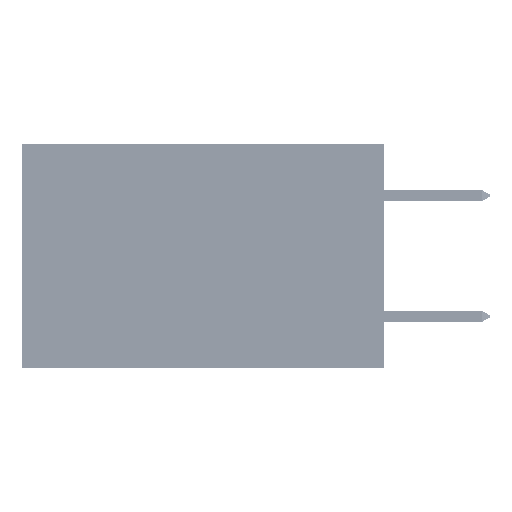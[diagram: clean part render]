
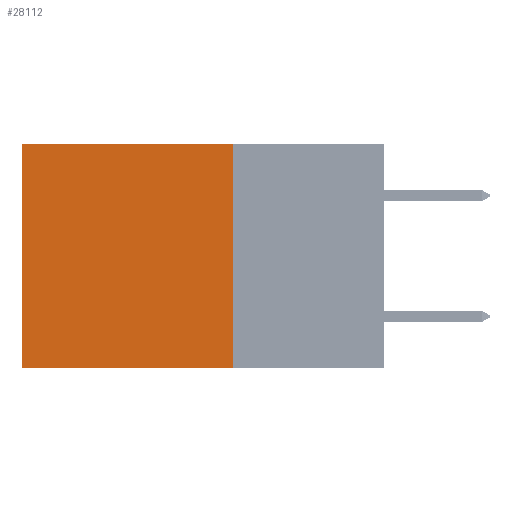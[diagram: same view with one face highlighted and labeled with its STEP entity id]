
A CAD part, left-side view. The second image highlights one B-rep face of the part: STEP entity #28112.
In plain terms, the highlighted planar face has unit normal (-1, 0, 0).
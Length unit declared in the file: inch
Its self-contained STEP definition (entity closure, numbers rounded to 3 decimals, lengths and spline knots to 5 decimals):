
#1281 = CARTESIAN_POINT ( 'NONE',  ( 0.2875, 0.25, 0. ) ) ;
#1449 = VECTOR ( 'NONE', #10237, 39.37008 ) ;
#1700 = FACE_OUTER_BOUND ( 'NONE', #33100, .T. ) ;
#1906 = CARTESIAN_POINT ( 'NONE',  ( 0.2875, 0.25, 0. ) ) ;
#2276 = DIRECTION ( 'NONE',  ( 0., 1., 0. ) ) ;
#2353 = EDGE_CURVE ( 'NONE', #35352, #40141, #32204, .T. ) ;
#5336 = ORIENTED_EDGE ( 'NONE', *, *, #24309, .F. ) ;
#5429 = DIRECTION ( 'NONE',  ( 0., 0., -1. ) ) ;
#9925 = VECTOR ( 'NONE', #2276, 39.37008 ) ;
#10237 = DIRECTION ( 'NONE',  ( 0., 0., -1. ) ) ;
#12402 = ORIENTED_EDGE ( 'NONE', *, *, #31972, .T. ) ;
#12416 = CARTESIAN_POINT ( 'NONE',  ( 0.2875, 0.6, 0. ) ) ;
#12793 = VERTEX_POINT ( 'NONE', #1906 ) ;
#14667 = CARTESIAN_POINT ( 'NONE',  ( 0.2875, 0.6, -0.37 ) ) ;
#14896 = CARTESIAN_POINT ( 'NONE',  ( 0.2875, 0.25, 0. ) ) ;
#17200 = PLANE ( 'NONE',  #48892 ) ;
#18864 = DIRECTION ( 'NONE',  ( 0., 1., 0. ) ) ;
#20450 = LINE ( 'NONE', #37939, #40270 ) ;
#23690 = LINE ( 'NONE', #29951, #1449 ) ;
#24309 = EDGE_CURVE ( 'NONE', #12793, #35352, #23690, .T. ) ;
#25764 = LINE ( 'NONE', #14896, #45591 ) ;
#28112 = ADVANCED_FACE ( 'NONE', ( #1700 ), #17200, .F. ) ;
#28723 = EDGE_CURVE ( 'NONE', #12793, #43951, #25764, .T. ) ;
#29095 = DIRECTION ( 'NONE',  ( 1., 0., 0. ) ) ;
#29689 = ORIENTED_EDGE ( 'NONE', *, *, #2353, .F. ) ;
#29951 = CARTESIAN_POINT ( 'NONE',  ( 0.2875, 0.25, 0. ) ) ;
#31972 = EDGE_CURVE ( 'NONE', #43951, #40141, #20450, .T. ) ;
#32204 = LINE ( 'NONE', #45708, #9925 ) ;
#33100 = EDGE_LOOP ( 'NONE', ( #12402, #29689, #5336, #33393 ) ) ;
#33393 = ORIENTED_EDGE ( 'NONE', *, *, #28723, .T. ) ;
#35352 = VERTEX_POINT ( 'NONE', #46713 ) ;
#37939 = CARTESIAN_POINT ( 'NONE',  ( 0.2875, 0.6, 0. ) ) ;
#40141 = VERTEX_POINT ( 'NONE', #14667 ) ;
#40270 = VECTOR ( 'NONE', #41945, 39.37008 ) ;
#41945 = DIRECTION ( 'NONE',  ( 0., 0., -1. ) ) ;
#43951 = VERTEX_POINT ( 'NONE', #12416 ) ;
#45591 = VECTOR ( 'NONE', #18864, 39.37008 ) ;
#45708 = CARTESIAN_POINT ( 'NONE',  ( 0.2875, 0.25, -0.37 ) ) ;
#46713 = CARTESIAN_POINT ( 'NONE',  ( 0.2875, 0.25, -0.37 ) ) ;
#48892 = AXIS2_PLACEMENT_3D ( 'NONE', #1281, #29095, #5429 ) ;
